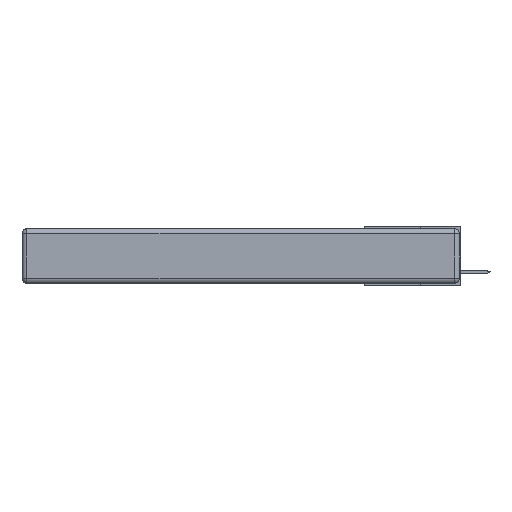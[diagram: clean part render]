
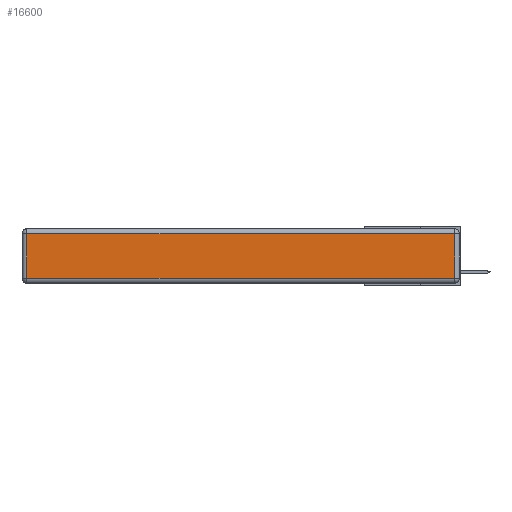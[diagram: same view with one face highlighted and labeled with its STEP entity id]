
A CAD part, left-side view. The second image highlights one B-rep face of the part: STEP entity #16600.
In plain terms, the highlighted planar face has unit normal (-1, 0, 0).
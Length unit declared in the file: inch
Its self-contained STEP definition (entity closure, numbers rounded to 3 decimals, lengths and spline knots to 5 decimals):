
#862 = CARTESIAN_POINT ( 'NONE',  ( 0., 2.72, -0.313 ) ) ;
#1702 = LINE ( 'NONE', #21077, #5283 ) ;
#2874 = EDGE_CURVE ( 'NONE', #21402, #22597, #23856, .T. ) ;
#3053 = VECTOR ( 'NONE', #21117, 39.37008 ) ;
#4084 = CARTESIAN_POINT ( 'NONE',  ( 0., 2.72, -0.343 ) ) ;
#4167 = DIRECTION ( 'NONE',  ( 0., 0., -1. ) ) ;
#4398 = CARTESIAN_POINT ( 'NONE',  ( 0., 0., -0.313 ) ) ;
#5073 = ORIENTED_EDGE ( 'NONE', *, *, #21081, .T. ) ;
#5264 = ORIENTED_EDGE ( 'NONE', *, *, #16367, .T. ) ;
#5283 = VECTOR ( 'NONE', #25186, 39.37008 ) ;
#5966 = LINE ( 'NONE', #25409, #3053 ) ;
#7296 = CARTESIAN_POINT ( 'NONE',  ( 0., 0.03, -0.03 ) ) ;
#9031 = VERTEX_POINT ( 'NONE', #7296 ) ;
#9676 = CARTESIAN_POINT ( 'NONE',  ( 0., 0., -0.343 ) ) ;
#10424 = EDGE_CURVE ( 'NONE', #22597, #19178, #11609, .T. ) ;
#11609 = LINE ( 'NONE', #4398, #15504 ) ;
#14660 = FACE_OUTER_BOUND ( 'NONE', #24610, .T. ) ;
#14818 = AXIS2_PLACEMENT_3D ( 'NONE', #9676, #20161, #25994 ) ;
#15165 = VECTOR ( 'NONE', #4167, 39.37008 ) ;
#15504 = VECTOR ( 'NONE', #20947, 39.37008 ) ;
#16089 = ORIENTED_EDGE ( 'NONE', *, *, #10424, .T. ) ;
#16367 = EDGE_CURVE ( 'NONE', #19178, #9031, #1702, .T. ) ;
#16600 = ADVANCED_FACE ( 'NONE', ( #14660 ), #22054, .T. ) ;
#18270 = CARTESIAN_POINT ( 'NONE',  ( 0., 2.72, -0.03 ) ) ;
#19018 = ORIENTED_EDGE ( 'NONE', *, *, #2874, .T. ) ;
#19178 = VERTEX_POINT ( 'NONE', #24618 ) ;
#20161 = DIRECTION ( 'NONE',  ( -1., 0., 0. ) ) ;
#20947 = DIRECTION ( 'NONE',  ( 0., -1., 0. ) ) ;
#21077 = CARTESIAN_POINT ( 'NONE',  ( 0., 0.03, -0.343 ) ) ;
#21081 = EDGE_CURVE ( 'NONE', #9031, #21402, #5966, .T. ) ;
#21117 = DIRECTION ( 'NONE',  ( 0., 1., 0. ) ) ;
#21402 = VERTEX_POINT ( 'NONE', #18270 ) ;
#22054 = PLANE ( 'NONE',  #14818 ) ;
#22597 = VERTEX_POINT ( 'NONE', #862 ) ;
#23856 = LINE ( 'NONE', #4084, #15165 ) ;
#24610 = EDGE_LOOP ( 'NONE', ( #16089, #5264, #5073, #19018 ) ) ;
#24618 = CARTESIAN_POINT ( 'NONE',  ( 0., 0.03, -0.313 ) ) ;
#25186 = DIRECTION ( 'NONE',  ( 0., 0., 1. ) ) ;
#25409 = CARTESIAN_POINT ( 'NONE',  ( 0., 2.75, -0.03 ) ) ;
#25994 = DIRECTION ( 'NONE',  ( 0., 0., 1. ) ) ;
